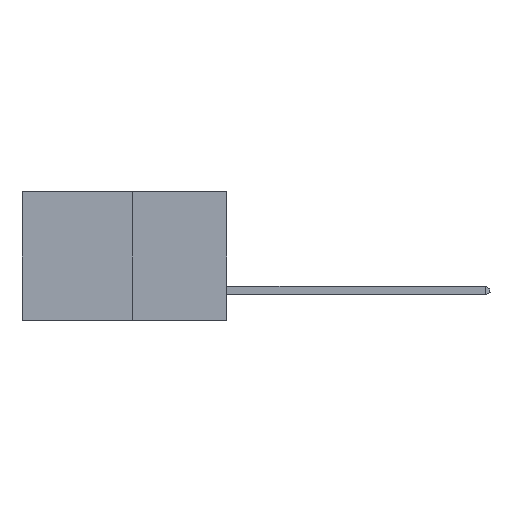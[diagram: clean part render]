
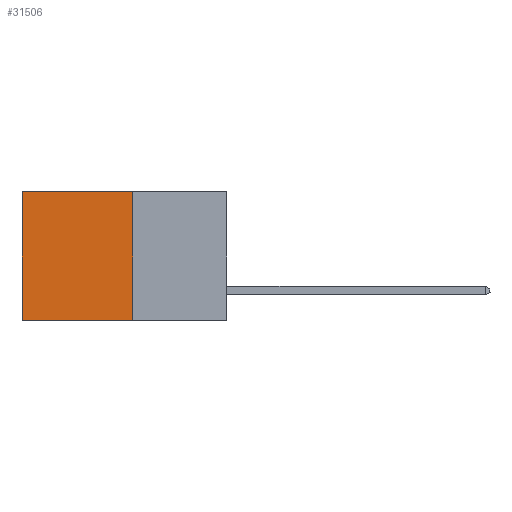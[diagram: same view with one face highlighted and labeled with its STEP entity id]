
A CAD part, left-side view. The second image highlights one B-rep face of the part: STEP entity #31506.
In plain terms, the highlighted planar face has unit normal (-1, 0, 0).
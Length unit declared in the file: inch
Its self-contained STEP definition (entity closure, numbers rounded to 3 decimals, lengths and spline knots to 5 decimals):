
#2010 = ORIENTED_EDGE ( 'NONE', *, *, #26471, .F. ) ;
#2232 = VERTEX_POINT ( 'NONE', #23701 ) ;
#2894 = EDGE_CURVE ( 'NONE', #7631, #2232, #16156, .T. ) ;
#3484 = VECTOR ( 'NONE', #4008, 39.37008 ) ;
#4008 = DIRECTION ( 'NONE',  ( 0., 1., 0. ) ) ;
#5216 = EDGE_CURVE ( 'NONE', #25729, #31927, #24679, .T. ) ;
#5728 = CARTESIAN_POINT ( 'NONE',  ( 0.277, 0.27, 0. ) ) ;
#5796 = CARTESIAN_POINT ( 'NONE',  ( 0.277, 0.27, 0. ) ) ;
#5843 = VECTOR ( 'NONE', #10920, 39.37008 ) ;
#6794 = FACE_OUTER_BOUND ( 'NONE', #21621, .T. ) ;
#7631 = VERTEX_POINT ( 'NONE', #5796 ) ;
#7643 = AXIS2_PLACEMENT_3D ( 'NONE', #27739, #14951, #32864 ) ;
#7781 = ORIENTED_EDGE ( 'NONE', *, *, #5216, .F. ) ;
#8342 = CARTESIAN_POINT ( 'NONE',  ( 0.277, 0.59, -0.37 ) ) ;
#8924 = DIRECTION ( 'NONE',  ( 0., 0., -1. ) ) ;
#9324 = VECTOR ( 'NONE', #10855, 39.37008 ) ;
#10855 = DIRECTION ( 'NONE',  ( 0., 1., 0. ) ) ;
#10920 = DIRECTION ( 'NONE',  ( 0., 0., -1. ) ) ;
#11241 = CARTESIAN_POINT ( 'NONE',  ( 0.277, 0.27, -0.37 ) ) ;
#14951 = DIRECTION ( 'NONE',  ( 1., 0., 0. ) ) ;
#16156 = LINE ( 'NONE', #5728, #9324 ) ;
#19450 = LINE ( 'NONE', #8342, #5843 ) ;
#20008 = LINE ( 'NONE', #24309, #27631 ) ;
#21224 = ORIENTED_EDGE ( 'NONE', *, *, #2894, .T. ) ;
#21621 = EDGE_LOOP ( 'NONE', ( #30392, #7781, #2010, #21224 ) ) ;
#21668 = CARTESIAN_POINT ( 'NONE',  ( 0.277, 0.59, -0.37 ) ) ;
#23115 = EDGE_CURVE ( 'NONE', #2232, #31927, #19450, .T. ) ;
#23701 = CARTESIAN_POINT ( 'NONE',  ( 0.277, 0.59, 0. ) ) ;
#24309 = CARTESIAN_POINT ( 'NONE',  ( 0.277, 0.27, -0.37 ) ) ;
#24679 = LINE ( 'NONE', #29502, #3484 ) ;
#25729 = VERTEX_POINT ( 'NONE', #11241 ) ;
#26471 = EDGE_CURVE ( 'NONE', #7631, #25729, #20008, .T. ) ;
#27631 = VECTOR ( 'NONE', #8924, 39.37008 ) ;
#27739 = CARTESIAN_POINT ( 'NONE',  ( 0.277, 0.27, -0.37 ) ) ;
#29502 = CARTESIAN_POINT ( 'NONE',  ( 0.277, 0.27, -0.37 ) ) ;
#30286 = PLANE ( 'NONE',  #7643 ) ;
#30392 = ORIENTED_EDGE ( 'NONE', *, *, #23115, .T. ) ;
#31506 = ADVANCED_FACE ( 'NONE', ( #6794 ), #30286, .F. ) ;
#31927 = VERTEX_POINT ( 'NONE', #21668 ) ;
#32864 = DIRECTION ( 'NONE',  ( 0., 0., -1. ) ) ;
